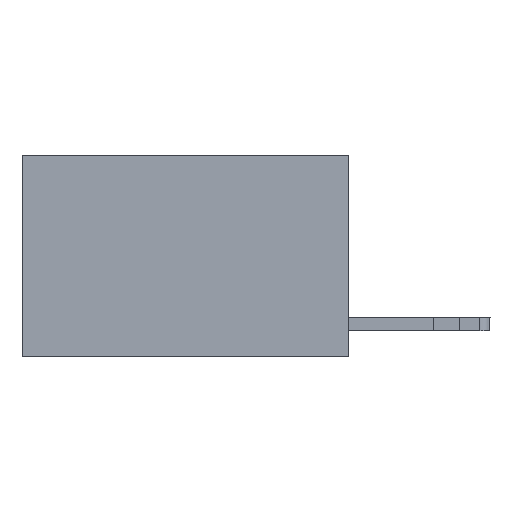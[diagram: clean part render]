
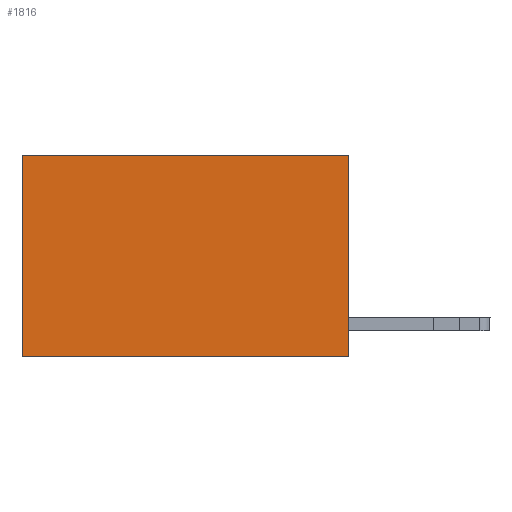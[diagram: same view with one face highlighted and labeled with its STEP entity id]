
A CAD part, left-side view. The second image highlights one B-rep face of the part: STEP entity #1816.
In plain terms, the highlighted planar face has unit normal (-1, 0, 0).
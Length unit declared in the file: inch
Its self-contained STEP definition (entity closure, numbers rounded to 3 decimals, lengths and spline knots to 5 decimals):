
#436 = CARTESIAN_POINT ( 'NONE',  ( 0.2625, 0., 0. ) ) ;
#882 = DIRECTION ( 'NONE',  ( 1., 0., 0. ) ) ;
#1256 = DIRECTION ( 'NONE',  ( 0., 1., 0. ) ) ;
#1703 = VECTOR ( 'NONE', #2267, 39.37008 ) ;
#1816 = ADVANCED_FACE ( 'NONE', ( #6567 ), #9803, .F. ) ;
#2267 = DIRECTION ( 'NONE',  ( 0., 0., -1. ) ) ;
#2683 = EDGE_LOOP ( 'NONE', ( #21143, #11047, #12743, #16284 ) ) ;
#3559 = EDGE_CURVE ( 'NONE', #17189, #19482, #7565, .T. ) ;
#4831 = CARTESIAN_POINT ( 'NONE',  ( 0.2625, 0., -0.37 ) ) ;
#6338 = CARTESIAN_POINT ( 'NONE',  ( 0.2625, 0., 0. ) ) ;
#6567 = FACE_OUTER_BOUND ( 'NONE', #2683, .T. ) ;
#6691 = CARTESIAN_POINT ( 'NONE',  ( 0.2625, 0., -0.37 ) ) ;
#7565 = LINE ( 'NONE', #436, #11677 ) ;
#8047 = CARTESIAN_POINT ( 'NONE',  ( 0.2625, 0., 0. ) ) ;
#8655 = AXIS2_PLACEMENT_3D ( 'NONE', #8047, #882, #22154 ) ;
#9173 = LINE ( 'NONE', #6691, #9715 ) ;
#9715 = VECTOR ( 'NONE', #1256, 39.37008 ) ;
#9803 = PLANE ( 'NONE',  #8655 ) ;
#10365 = EDGE_CURVE ( 'NONE', #12103, #21835, #9173, .T. ) ;
#10512 = EDGE_CURVE ( 'NONE', #19482, #21835, #16153, .T. ) ;
#11047 = ORIENTED_EDGE ( 'NONE', *, *, #10365, .F. ) ;
#11064 = CARTESIAN_POINT ( 'NONE',  ( 0.2625, 0., 0. ) ) ;
#11677 = VECTOR ( 'NONE', #12766, 39.37008 ) ;
#12103 = VERTEX_POINT ( 'NONE', #4831 ) ;
#12743 = ORIENTED_EDGE ( 'NONE', *, *, #17659, .F. ) ;
#12766 = DIRECTION ( 'NONE',  ( 0., 1., 0. ) ) ;
#15226 = LINE ( 'NONE', #11064, #1703 ) ;
#16153 = LINE ( 'NONE', #17695, #19692 ) ;
#16284 = ORIENTED_EDGE ( 'NONE', *, *, #3559, .T. ) ;
#17189 = VERTEX_POINT ( 'NONE', #6338 ) ;
#17616 = DIRECTION ( 'NONE',  ( 0., 0., -1. ) ) ;
#17659 = EDGE_CURVE ( 'NONE', #17189, #12103, #15226, .T. ) ;
#17695 = CARTESIAN_POINT ( 'NONE',  ( 0.2625, 0.6, 0. ) ) ;
#19335 = CARTESIAN_POINT ( 'NONE',  ( 0.2625, 0.6, 0. ) ) ;
#19482 = VERTEX_POINT ( 'NONE', #19335 ) ;
#19692 = VECTOR ( 'NONE', #17616, 39.37008 ) ;
#20538 = CARTESIAN_POINT ( 'NONE',  ( 0.2625, 0.6, -0.37 ) ) ;
#21143 = ORIENTED_EDGE ( 'NONE', *, *, #10512, .T. ) ;
#21835 = VERTEX_POINT ( 'NONE', #20538 ) ;
#22154 = DIRECTION ( 'NONE',  ( 0., 0., -1. ) ) ;
